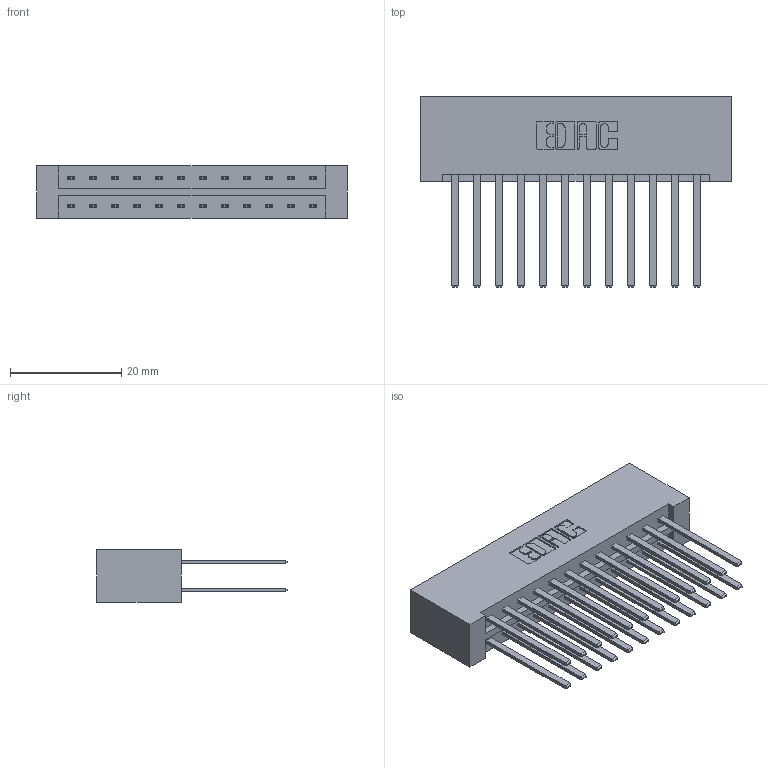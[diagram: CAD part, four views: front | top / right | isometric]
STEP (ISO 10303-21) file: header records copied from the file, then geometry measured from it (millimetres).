
FILE_DESCRIPTION (( 'STEP AP203' ), '1' );
FILE_NAME ('333-024-544-201.STEP', '2018-08-02T11:26:36', ( '' ), ( '' ), 'SwSTEP 2.0', 'SolidWorks 2016', '' );
FILE_SCHEMA (( 'CONFIG_CONTROL_DESIGN' ));
Length unit declared in the file: inch
Products named in the file (3): 333 Part_Lugless; 345-292-001_345-293-144; 333-024-544-201
Assembly tree (25 placements, depth 2):
  333-024-544-201
    333 Part_Lugless
    345-292-001_345-293-144  x24
Bounding box: 55.8 x 34.3 x 9.4 mm (x, y, z)
Volume: 6385.4 mm3; surface area: 8334.3 mm2
Topology: 25 solids, 25 shells, 1210 faces, 3575 edges, 2350 vertices
Faces by surface type: plane 834, cylinder 376
Entity records: 11139 total; most frequent: CARTESIAN_POINT 1878, ORIENTED_EDGE 1814, DIRECTION 1647, EDGE_CURVE 907, VECTOR 791, LINE 791, VERTEX_POINT 602, AXIS2_PLACEMENT_3D 428
